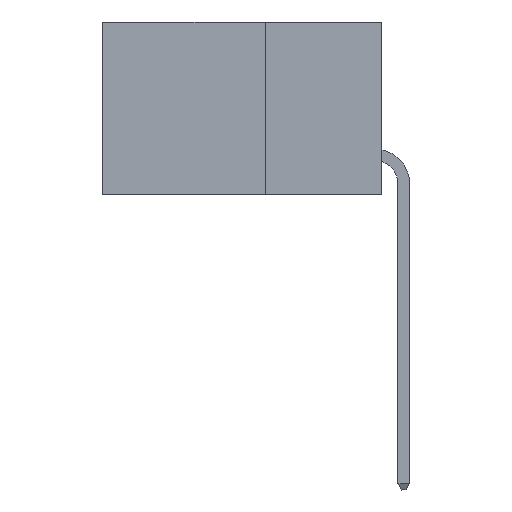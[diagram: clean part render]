
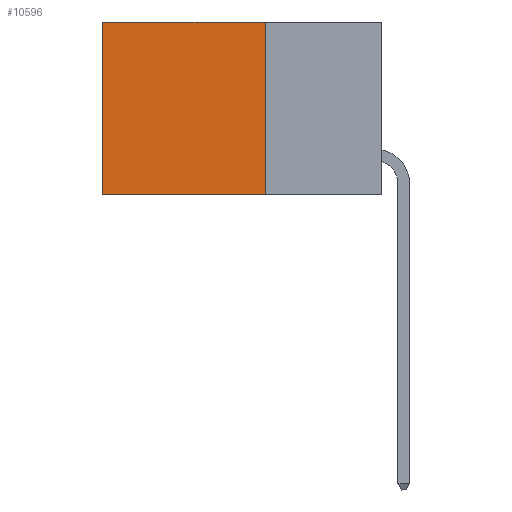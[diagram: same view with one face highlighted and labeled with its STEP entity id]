
A CAD part, left-side view. The second image highlights one B-rep face of the part: STEP entity #10596.
In plain terms, the highlighted planar face has unit normal (-1, 0, 0).
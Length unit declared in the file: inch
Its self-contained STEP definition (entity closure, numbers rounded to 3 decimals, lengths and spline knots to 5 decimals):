
#916 = VECTOR ( 'NONE', #14236, 39.37008 ) ;
#1117 = VECTOR ( 'NONE', #6870, 39.37008 ) ;
#1320 = CARTESIAN_POINT ( 'NONE',  ( 0.2875, 0.25, -0.37 ) ) ;
#1653 = ORIENTED_EDGE ( 'NONE', *, *, #13076, .F. ) ;
#2008 = VERTEX_POINT ( 'NONE', #7353 ) ;
#2560 = CARTESIAN_POINT ( 'NONE',  ( 0.2875, 0.6, 0. ) ) ;
#2650 = DIRECTION ( 'NONE',  ( 0., 1., 0. ) ) ;
#3489 = DIRECTION ( 'NONE',  ( 0., 0., -1. ) ) ;
#3493 = CARTESIAN_POINT ( 'NONE',  ( 0.2875, 0.25, 0. ) ) ;
#3533 = AXIS2_PLACEMENT_3D ( 'NONE', #15066, #11288, #3489 ) ;
#3872 = ORIENTED_EDGE ( 'NONE', *, *, #12386, .F. ) ;
#5139 = VERTEX_POINT ( 'NONE', #3493 ) ;
#5335 = ORIENTED_EDGE ( 'NONE', *, *, #7155, .T. ) ;
#6870 = DIRECTION ( 'NONE',  ( 0., 0., -1. ) ) ;
#7155 = EDGE_CURVE ( 'NONE', #5139, #9171, #8537, .T. ) ;
#7353 = CARTESIAN_POINT ( 'NONE',  ( 0.2875, 0.25, -0.37 ) ) ;
#8330 = LINE ( 'NONE', #2560, #916 ) ;
#8537 = LINE ( 'NONE', #13124, #11553 ) ;
#8678 = VERTEX_POINT ( 'NONE', #16054 ) ;
#8769 = EDGE_LOOP ( 'NONE', ( #16442, #1653, #3872, #5335 ) ) ;
#9171 = VERTEX_POINT ( 'NONE', #9545 ) ;
#9545 = CARTESIAN_POINT ( 'NONE',  ( 0.2875, 0.6, 0. ) ) ;
#10596 = ADVANCED_FACE ( 'NONE', ( #14989 ), #16351, .F. ) ;
#11288 = DIRECTION ( 'NONE',  ( 1., 0., 0. ) ) ;
#11545 = LINE ( 'NONE', #12070, #1117 ) ;
#11553 = VECTOR ( 'NONE', #11868, 39.37008 ) ;
#11868 = DIRECTION ( 'NONE',  ( 0., 1., 0. ) ) ;
#12070 = CARTESIAN_POINT ( 'NONE',  ( 0.2875, 0.25, 0. ) ) ;
#12157 = EDGE_CURVE ( 'NONE', #9171, #8678, #8330, .T. ) ;
#12386 = EDGE_CURVE ( 'NONE', #5139, #2008, #11545, .T. ) ;
#13076 = EDGE_CURVE ( 'NONE', #2008, #8678, #15317, .T. ) ;
#13124 = CARTESIAN_POINT ( 'NONE',  ( 0.2875, 0.25, 0. ) ) ;
#14236 = DIRECTION ( 'NONE',  ( 0., 0., -1. ) ) ;
#14927 = VECTOR ( 'NONE', #2650, 39.37008 ) ;
#14989 = FACE_OUTER_BOUND ( 'NONE', #8769, .T. ) ;
#15066 = CARTESIAN_POINT ( 'NONE',  ( 0.2875, 0.25, 0. ) ) ;
#15317 = LINE ( 'NONE', #1320, #14927 ) ;
#16054 = CARTESIAN_POINT ( 'NONE',  ( 0.2875, 0.6, -0.37 ) ) ;
#16351 = PLANE ( 'NONE',  #3533 ) ;
#16442 = ORIENTED_EDGE ( 'NONE', *, *, #12157, .T. ) ;
